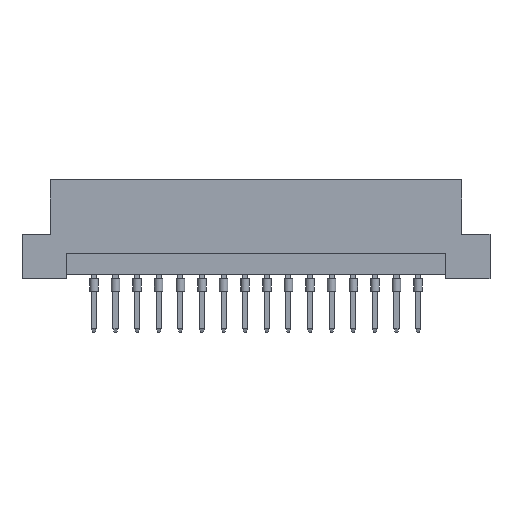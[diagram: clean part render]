
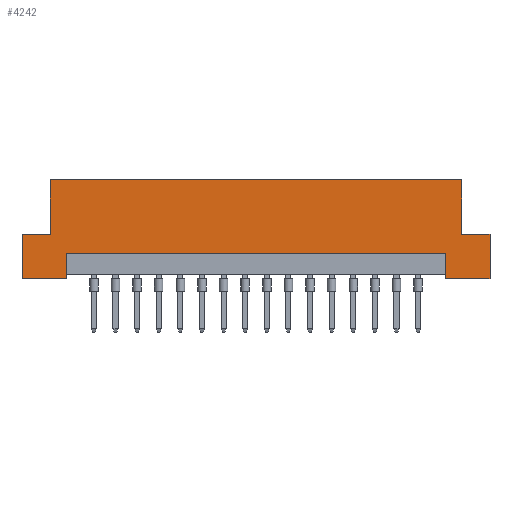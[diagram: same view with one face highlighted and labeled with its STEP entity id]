
A CAD part, front view. The second image highlights one B-rep face of the part: STEP entity #4242.
In plain terms, the highlighted planar face has unit normal (0, -1, 0).
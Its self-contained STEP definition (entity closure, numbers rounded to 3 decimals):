
#10 = CARTESIAN_POINT ( 'NONE',  ( -27.5, 0., 11.6 ) ) ;
#99 = DIRECTION ( 'NONE',  ( 0., 0., 1. ) ) ;
#113 = CARTESIAN_POINT ( 'NONE',  ( 27.5, 0., 0. ) ) ;
#355 = ORIENTED_EDGE ( 'NONE', *, *, #8578, .F. ) ;
#503 = LINE ( 'NONE', #5563, #7410 ) ;
#636 = VECTOR ( 'NONE', #3740, 1000. ) ;
#656 = CARTESIAN_POINT ( 'NONE',  ( -22.3, 0., 2.9 ) ) ;
#743 = FACE_OUTER_BOUND ( 'NONE', #7514, .T. ) ;
#908 = VERTEX_POINT ( 'NONE', #6646 ) ;
#1002 = CARTESIAN_POINT ( 'NONE',  ( -27.5, 0., 0. ) ) ;
#1006 = CARTESIAN_POINT ( 'NONE',  ( 27.5, 0., 5.2 ) ) ;
#1160 = DIRECTION ( 'NONE',  ( 1., 0., 0. ) ) ;
#1202 = CARTESIAN_POINT ( 'NONE',  ( -24.2, 0., 11.6 ) ) ;
#1516 = DIRECTION ( 'NONE',  ( 0., 1., 0. ) ) ;
#1705 = PLANE ( 'NONE',  #5810 ) ;
#1803 = EDGE_CURVE ( 'NONE', #5546, #5282, #7209, .T. ) ;
#1847 = DIRECTION ( 'NONE',  ( 0., 0., -1. ) ) ;
#2497 = LINE ( 'NONE', #1002, #6100 ) ;
#2528 = EDGE_CURVE ( 'NONE', #5546, #5560, #8445, .T. ) ;
#2537 = LINE ( 'NONE', #5476, #5494 ) ;
#2869 = EDGE_CURVE ( 'NONE', #7537, #908, #2497, .T. ) ;
#3022 = ORIENTED_EDGE ( 'NONE', *, *, #5631, .T. ) ;
#3030 = CARTESIAN_POINT ( 'NONE',  ( -27.5, 0., 0. ) ) ;
#3153 = CARTESIAN_POINT ( 'NONE',  ( 24.2, 0., 11.6 ) ) ;
#3181 = CARTESIAN_POINT ( 'NONE',  ( -22.3, 0., 0.5 ) ) ;
#3367 = VERTEX_POINT ( 'NONE', #1006 ) ;
#3467 = VECTOR ( 'NONE', #1160, 1000. ) ;
#3478 = ORIENTED_EDGE ( 'NONE', *, *, #2869, .F. ) ;
#3486 = VERTEX_POINT ( 'NONE', #1202 ) ;
#3536 = CARTESIAN_POINT ( 'NONE',  ( 24.2, 0., 5.2 ) ) ;
#3740 = DIRECTION ( 'NONE',  ( 0., 0., -1. ) ) ;
#3925 = LINE ( 'NONE', #113, #636 ) ;
#3997 = EDGE_CURVE ( 'NONE', #3486, #4172, #2537, .T. ) ;
#4172 = VERTEX_POINT ( 'NONE', #3153 ) ;
#4242 = ADVANCED_FACE ( 'NONE', ( #743 ), #1705, .F. ) ;
#4394 = DIRECTION ( 'NONE',  ( -1., 0., 0. ) ) ;
#4441 = CARTESIAN_POINT ( 'NONE',  ( -27.5, 0., 0. ) ) ;
#4489 = LINE ( 'NONE', #4441, #8341 ) ;
#4522 = VERTEX_POINT ( 'NONE', #5846 ) ;
#4545 = VERTEX_POINT ( 'NONE', #3536 ) ;
#4550 = CARTESIAN_POINT ( 'NONE',  ( -24.2, 0., 5.2 ) ) ;
#4660 = ORIENTED_EDGE ( 'NONE', *, *, #5973, .F. ) ;
#4703 = EDGE_CURVE ( 'NONE', #5282, #8961, #5351, .T. ) ;
#5088 = CARTESIAN_POINT ( 'NONE',  ( 27.5, 0., 0. ) ) ;
#5155 = LINE ( 'NONE', #3030, #6533 ) ;
#5216 = LINE ( 'NONE', #4550, #5715 ) ;
#5282 = VERTEX_POINT ( 'NONE', #656 ) ;
#5284 = CARTESIAN_POINT ( 'NONE',  ( 22.3, 0., 0. ) ) ;
#5351 = LINE ( 'NONE', #3181, #5907 ) ;
#5379 = VECTOR ( 'NONE', #8848, 1000. ) ;
#5411 = CARTESIAN_POINT ( 'NONE',  ( -27.5, 0., 0. ) ) ;
#5423 = ORIENTED_EDGE ( 'NONE', *, *, #2528, .T. ) ;
#5476 = CARTESIAN_POINT ( 'NONE',  ( -27.5, 0., 11.6 ) ) ;
#5494 = VECTOR ( 'NONE', #8419, 1000. ) ;
#5495 = CARTESIAN_POINT ( 'NONE',  ( 27.5, 0., 5.2 ) ) ;
#5528 = EDGE_CURVE ( 'NONE', #3367, #8703, #3925, .T. ) ;
#5546 = VERTEX_POINT ( 'NONE', #6137 ) ;
#5552 = CARTESIAN_POINT ( 'NONE',  ( 22.3, 0., 0.5 ) ) ;
#5560 = VERTEX_POINT ( 'NONE', #5284 ) ;
#5563 = CARTESIAN_POINT ( 'NONE',  ( 24.2, 0., 5.2 ) ) ;
#5631 = EDGE_CURVE ( 'NONE', #4545, #4172, #503, .T. ) ;
#5715 = VECTOR ( 'NONE', #99, 1000. ) ;
#5721 = DIRECTION ( 'NONE',  ( 0., 0., 1. ) ) ;
#5810 = AXIS2_PLACEMENT_3D ( 'NONE', #10, #1516, #8891 ) ;
#5846 = CARTESIAN_POINT ( 'NONE',  ( -24.2, 0., 5.2 ) ) ;
#5907 = VECTOR ( 'NONE', #7607, 1000. ) ;
#5968 = DIRECTION ( 'NONE',  ( -1., 0., 0. ) ) ;
#5973 = EDGE_CURVE ( 'NONE', #4522, #3486, #5216, .T. ) ;
#6100 = VECTOR ( 'NONE', #5721, 1000. ) ;
#6119 = LINE ( 'NONE', #5495, #3467 ) ;
#6137 = CARTESIAN_POINT ( 'NONE',  ( 22.3, 0., 2.9 ) ) ;
#6160 = ORIENTED_EDGE ( 'NONE', *, *, #6360, .F. ) ;
#6360 = EDGE_CURVE ( 'NONE', #8703, #5560, #4489, .T. ) ;
#6475 = ORIENTED_EDGE ( 'NONE', *, *, #5528, .F. ) ;
#6533 = VECTOR ( 'NONE', #5968, 1000. ) ;
#6623 = CARTESIAN_POINT ( 'NONE',  ( 22.3, 0., 2.9 ) ) ;
#6646 = CARTESIAN_POINT ( 'NONE',  ( -27.5, 0., 5.2 ) ) ;
#7209 = LINE ( 'NONE', #6623, #5379 ) ;
#7410 = VECTOR ( 'NONE', #8456, 1000. ) ;
#7514 = EDGE_LOOP ( 'NONE', ( #8972, #5423, #6160, #6475, #8449, #3022, #9102, #4660, #355, #3478, #7586, #9331 ) ) ;
#7537 = VERTEX_POINT ( 'NONE', #5411 ) ;
#7586 = ORIENTED_EDGE ( 'NONE', *, *, #8478, .F. ) ;
#7607 = DIRECTION ( 'NONE',  ( 0., 0., -1. ) ) ;
#8024 = LINE ( 'NONE', #8840, #8086 ) ;
#8073 = DIRECTION ( 'NONE',  ( 1., 0., 0. ) ) ;
#8086 = VECTOR ( 'NONE', #8073, 1000. ) ;
#8180 = EDGE_CURVE ( 'NONE', #4545, #3367, #6119, .T. ) ;
#8254 = VECTOR ( 'NONE', #1847, 1000. ) ;
#8341 = VECTOR ( 'NONE', #4394, 1000. ) ;
#8419 = DIRECTION ( 'NONE',  ( 1., 0., 0. ) ) ;
#8445 = LINE ( 'NONE', #5552, #8254 ) ;
#8449 = ORIENTED_EDGE ( 'NONE', *, *, #8180, .F. ) ;
#8456 = DIRECTION ( 'NONE',  ( 0., 0., 1. ) ) ;
#8478 = EDGE_CURVE ( 'NONE', #8961, #7537, #5155, .T. ) ;
#8578 = EDGE_CURVE ( 'NONE', #908, #4522, #8024, .T. ) ;
#8703 = VERTEX_POINT ( 'NONE', #5088 ) ;
#8840 = CARTESIAN_POINT ( 'NONE',  ( -27.5, 0., 5.2 ) ) ;
#8848 = DIRECTION ( 'NONE',  ( -1., 0., 0. ) ) ;
#8891 = DIRECTION ( 'NONE',  ( 0., 0., 1. ) ) ;
#8961 = VERTEX_POINT ( 'NONE', #9176 ) ;
#8972 = ORIENTED_EDGE ( 'NONE', *, *, #1803, .F. ) ;
#9102 = ORIENTED_EDGE ( 'NONE', *, *, #3997, .F. ) ;
#9176 = CARTESIAN_POINT ( 'NONE',  ( -22.3, 0., 0. ) ) ;
#9331 = ORIENTED_EDGE ( 'NONE', *, *, #4703, .F. ) ;
